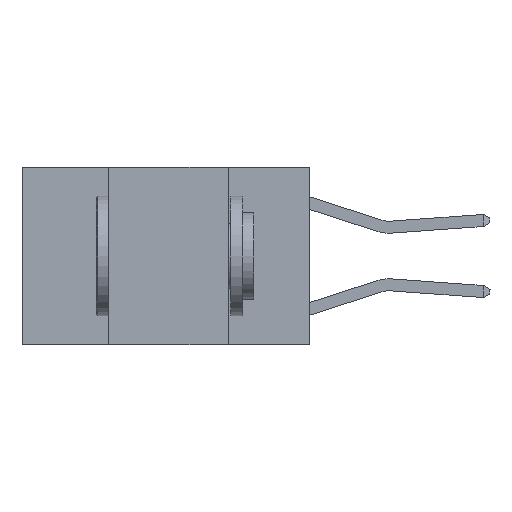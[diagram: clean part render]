
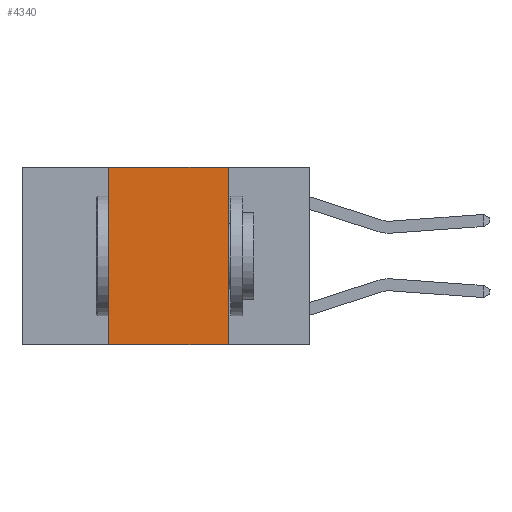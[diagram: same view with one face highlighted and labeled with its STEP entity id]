
A CAD part, left-side view. The second image highlights one B-rep face of the part: STEP entity #4340.
In plain terms, the highlighted planar face has unit normal (-1, 0, 0).
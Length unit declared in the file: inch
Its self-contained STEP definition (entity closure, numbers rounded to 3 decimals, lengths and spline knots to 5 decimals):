
#104 = FACE_OUTER_BOUND ( 'NONE', #11491, .T. ) ;
#217 = CARTESIAN_POINT ( 'NONE',  ( 0., 0.6, 0. ) ) ;
#337 = CARTESIAN_POINT ( 'NONE',  ( 0., 0.17, 0. ) ) ;
#448 = VECTOR ( 'NONE', #1539, 39.37008 ) ;
#477 = LINE ( 'NONE', #6035, #5036 ) ;
#480 = ORIENTED_EDGE ( 'NONE', *, *, #1162, .F. ) ;
#1100 = VECTOR ( 'NONE', #1137, 39.37008 ) ;
#1137 = DIRECTION ( 'NONE',  ( 0., -1., 0. ) ) ;
#1162 = EDGE_CURVE ( 'NONE', #11624, #7851, #477, .T. ) ;
#1539 = DIRECTION ( 'NONE',  ( 0., 0., 1. ) ) ;
#1789 = CARTESIAN_POINT ( 'NONE',  ( 0., 0.6, 0. ) ) ;
#2016 = DIRECTION ( 'NONE',  ( 0., -1., 0. ) ) ;
#2697 = DIRECTION ( 'NONE',  ( 0., 0., -1. ) ) ;
#4145 = CARTESIAN_POINT ( 'NONE',  ( 0., 0.17, -0.37 ) ) ;
#4340 = ADVANCED_FACE ( 'NONE', ( #104 ), #6308, .F. ) ;
#4643 = CARTESIAN_POINT ( 'NONE',  ( 0., 0.42, -0.37 ) ) ;
#5036 = VECTOR ( 'NONE', #10877, 39.37008 ) ;
#5461 = VECTOR ( 'NONE', #2016, 39.37008 ) ;
#5771 = ORIENTED_EDGE ( 'NONE', *, *, #9304, .F. ) ;
#6035 = CARTESIAN_POINT ( 'NONE',  ( 0., 0.17, 0. ) ) ;
#6161 = ORIENTED_EDGE ( 'NONE', *, *, #7674, .T. ) ;
#6308 = PLANE ( 'NONE',  #10057 ) ;
#6324 = VERTEX_POINT ( 'NONE', #4643 ) ;
#7674 = EDGE_CURVE ( 'NONE', #6324, #7851, #10256, .T. ) ;
#7772 = LINE ( 'NONE', #217, #1100 ) ;
#7851 = VERTEX_POINT ( 'NONE', #4145 ) ;
#7882 = ORIENTED_EDGE ( 'NONE', *, *, #11546, .F. ) ;
#8141 = DIRECTION ( 'NONE',  ( 1., 0., 0. ) ) ;
#8804 = CARTESIAN_POINT ( 'NONE',  ( 0., 0.42, 0. ) ) ;
#9304 = EDGE_CURVE ( 'NONE', #6324, #10426, #10081, .T. ) ;
#9567 = CARTESIAN_POINT ( 'NONE',  ( 0., 0.42, 0. ) ) ;
#10057 = AXIS2_PLACEMENT_3D ( 'NONE', #1789, #8141, #2697 ) ;
#10081 = LINE ( 'NONE', #8804, #448 ) ;
#10133 = CARTESIAN_POINT ( 'NONE',  ( 0., 0.6, -0.37 ) ) ;
#10256 = LINE ( 'NONE', #10133, #5461 ) ;
#10426 = VERTEX_POINT ( 'NONE', #9567 ) ;
#10877 = DIRECTION ( 'NONE',  ( 0., 0., -1. ) ) ;
#11491 = EDGE_LOOP ( 'NONE', ( #480, #7882, #5771, #6161 ) ) ;
#11546 = EDGE_CURVE ( 'NONE', #10426, #11624, #7772, .T. ) ;
#11624 = VERTEX_POINT ( 'NONE', #337 ) ;
